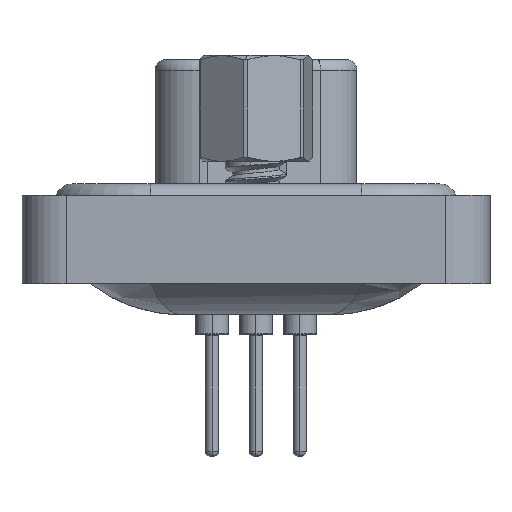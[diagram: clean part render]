
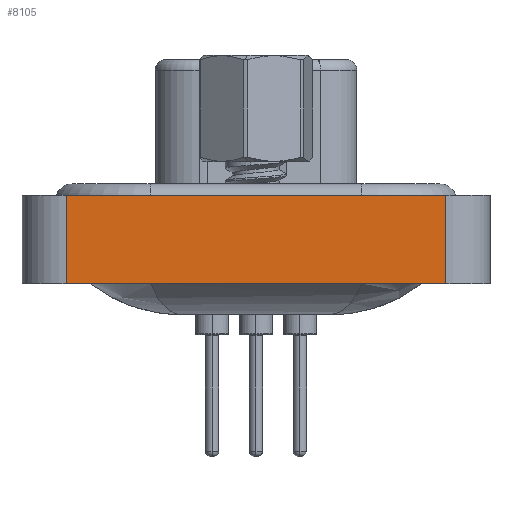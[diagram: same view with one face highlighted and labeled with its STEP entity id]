
A CAD part, left-side view. The second image highlights one B-rep face of the part: STEP entity #8105.
In plain terms, the highlighted planar face has unit normal (-1, 0, 0).
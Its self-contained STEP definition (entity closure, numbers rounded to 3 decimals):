
#1340 = ORIENTED_EDGE ( 'NONE', *, *, #8668, .T. ) ;
#2435 = PLANE ( 'NONE',  #2914 ) ;
#2575 = LINE ( 'NONE', #10577, #7726 ) ;
#2914 = AXIS2_PLACEMENT_3D ( 'NONE', #20723, #23567, #31353 ) ;
#4015 = CARTESIAN_POINT ( 'NONE',  ( -7.35, 8.55, -3.6 ) ) ;
#4395 = CARTESIAN_POINT ( 'NONE',  ( -7.35, -8.55, -3.6 ) ) ;
#4644 = EDGE_LOOP ( 'NONE', ( #1340, #8805, #20943, #7361 ) ) ;
#4733 = LINE ( 'NONE', #18063, #19945 ) ;
#5883 = VERTEX_POINT ( 'NONE', #7666 ) ;
#6110 = DIRECTION ( 'NONE',  ( 0., -1., 0. ) ) ;
#6607 = VERTEX_POINT ( 'NONE', #10648 ) ;
#7361 = ORIENTED_EDGE ( 'NONE', *, *, #16297, .T. ) ;
#7666 = CARTESIAN_POINT ( 'NONE',  ( -7.35, -8.55, 0.4 ) ) ;
#7726 = VECTOR ( 'NONE', #26701, 1000. ) ;
#8014 = EDGE_CURVE ( 'NONE', #10850, #5883, #4733, .T. ) ;
#8105 = ADVANCED_FACE ( 'NONE', ( #34344 ), #2435, .T. ) ;
#8668 = EDGE_CURVE ( 'NONE', #15184, #5883, #2575, .T. ) ;
#8805 = ORIENTED_EDGE ( 'NONE', *, *, #8014, .F. ) ;
#10577 = CARTESIAN_POINT ( 'NONE',  ( -7.35, -8.55, -3.6 ) ) ;
#10648 = CARTESIAN_POINT ( 'NONE',  ( -7.35, 8.55, -3.6 ) ) ;
#10850 = VERTEX_POINT ( 'NONE', #24049 ) ;
#11452 = LINE ( 'NONE', #27744, #16577 ) ;
#15184 = VERTEX_POINT ( 'NONE', #4395 ) ;
#16297 = EDGE_CURVE ( 'NONE', #6607, #15184, #11452, .T. ) ;
#16577 = VECTOR ( 'NONE', #6110, 1000. ) ;
#18063 = CARTESIAN_POINT ( 'NONE',  ( -7.35, -8.55, 0.4 ) ) ;
#19945 = VECTOR ( 'NONE', #20888, 1000. ) ;
#20723 = CARTESIAN_POINT ( 'NONE',  ( -7.35, -8.55, -3.6 ) ) ;
#20888 = DIRECTION ( 'NONE',  ( 0., -1., 0. ) ) ;
#20943 = ORIENTED_EDGE ( 'NONE', *, *, #21917, .F. ) ;
#21917 = EDGE_CURVE ( 'NONE', #6607, #10850, #31332, .T. ) ;
#23567 = DIRECTION ( 'NONE',  ( -1., 0., 0. ) ) ;
#24049 = CARTESIAN_POINT ( 'NONE',  ( -7.35, 8.55, 0.4 ) ) ;
#26701 = DIRECTION ( 'NONE',  ( 0., 0., 1. ) ) ;
#27744 = CARTESIAN_POINT ( 'NONE',  ( -7.35, -8.55, -3.6 ) ) ;
#28128 = VECTOR ( 'NONE', #31157, 1000. ) ;
#31157 = DIRECTION ( 'NONE',  ( 0., 0., 1. ) ) ;
#31332 = LINE ( 'NONE', #4015, #28128 ) ;
#31353 = DIRECTION ( 'NONE',  ( 0., 0., 1. ) ) ;
#34344 = FACE_OUTER_BOUND ( 'NONE', #4644, .T. ) ;
